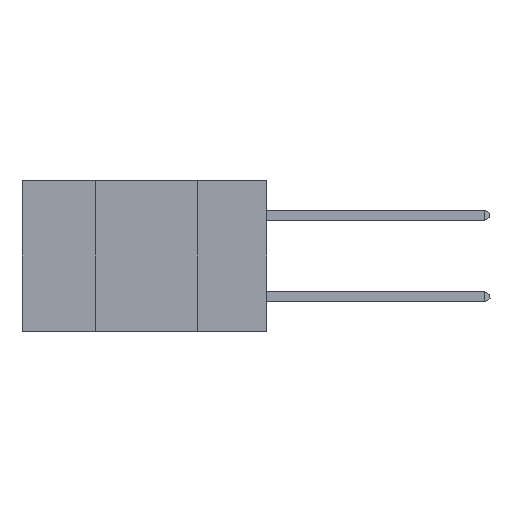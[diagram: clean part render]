
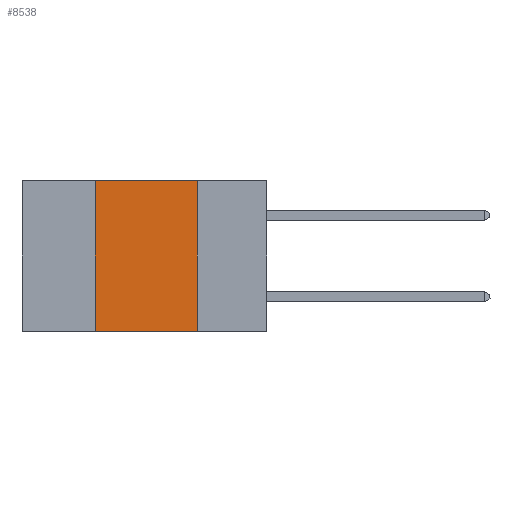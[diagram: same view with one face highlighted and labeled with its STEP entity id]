
A CAD part, left-side view. The second image highlights one B-rep face of the part: STEP entity #8538.
In plain terms, the highlighted planar face has unit normal (-1, 0, 0).
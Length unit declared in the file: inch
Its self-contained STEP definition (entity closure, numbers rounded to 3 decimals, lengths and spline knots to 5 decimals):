
#31 = VECTOR ( 'NONE', #13116, 39.37008 ) ;
#788 = AXIS2_PLACEMENT_3D ( 'NONE', #8922, #10707, #10391 ) ;
#3715 = CARTESIAN_POINT ( 'NONE',  ( 0., 0.6, 0. ) ) ;
#4338 = CARTESIAN_POINT ( 'NONE',  ( 0., 0.6, -0.37 ) ) ;
#4341 = ORIENTED_EDGE ( 'NONE', *, *, #21345, .F. ) ;
#4663 = CARTESIAN_POINT ( 'NONE',  ( 0., 0.17, 0. ) ) ;
#5050 = EDGE_CURVE ( 'NONE', #6617, #7502, #19262, .T. ) ;
#5652 = CARTESIAN_POINT ( 'NONE',  ( 0., 0.42, -0.37 ) ) ;
#6617 = VERTEX_POINT ( 'NONE', #5652 ) ;
#7502 = VERTEX_POINT ( 'NONE', #14924 ) ;
#8379 = CARTESIAN_POINT ( 'NONE',  ( 0., 0.17, 0. ) ) ;
#8538 = ADVANCED_FACE ( 'NONE', ( #9064 ), #19614, .F. ) ;
#8922 = CARTESIAN_POINT ( 'NONE',  ( 0., 0.6, 0. ) ) ;
#9064 = FACE_OUTER_BOUND ( 'NONE', #20073, .T. ) ;
#10391 = DIRECTION ( 'NONE',  ( 0., 0., -1. ) ) ;
#10675 = CARTESIAN_POINT ( 'NONE',  ( 0., 0.42, 0. ) ) ;
#10707 = DIRECTION ( 'NONE',  ( 1., 0., 0. ) ) ;
#12157 = LINE ( 'NONE', #3715, #15767 ) ;
#12745 = VERTEX_POINT ( 'NONE', #10675 ) ;
#13116 = DIRECTION ( 'NONE',  ( 0., 0., 1. ) ) ;
#13186 = DIRECTION ( 'NONE',  ( 0., -1., 0. ) ) ;
#13650 = EDGE_CURVE ( 'NONE', #6617, #12745, #14254, .T. ) ;
#14064 = ORIENTED_EDGE ( 'NONE', *, *, #5050, .T. ) ;
#14254 = LINE ( 'NONE', #22060, #31 ) ;
#14924 = CARTESIAN_POINT ( 'NONE',  ( 0., 0.17, -0.37 ) ) ;
#15291 = DIRECTION ( 'NONE',  ( 0., 0., -1. ) ) ;
#15767 = VECTOR ( 'NONE', #17992, 39.37008 ) ;
#17992 = DIRECTION ( 'NONE',  ( 0., -1., 0. ) ) ;
#18139 = VECTOR ( 'NONE', #13186, 39.37008 ) ;
#19262 = LINE ( 'NONE', #4338, #18139 ) ;
#19334 = EDGE_CURVE ( 'NONE', #12745, #21043, #12157, .T. ) ;
#19614 = PLANE ( 'NONE',  #788 ) ;
#19688 = ORIENTED_EDGE ( 'NONE', *, *, #19334, .F. ) ;
#20073 = EDGE_LOOP ( 'NONE', ( #4341, #19688, #23006, #14064 ) ) ;
#21043 = VERTEX_POINT ( 'NONE', #8379 ) ;
#21091 = VECTOR ( 'NONE', #15291, 39.37008 ) ;
#21345 = EDGE_CURVE ( 'NONE', #21043, #7502, #21638, .T. ) ;
#21638 = LINE ( 'NONE', #4663, #21091 ) ;
#22060 = CARTESIAN_POINT ( 'NONE',  ( 0., 0.42, 0. ) ) ;
#23006 = ORIENTED_EDGE ( 'NONE', *, *, #13650, .F. ) ;
